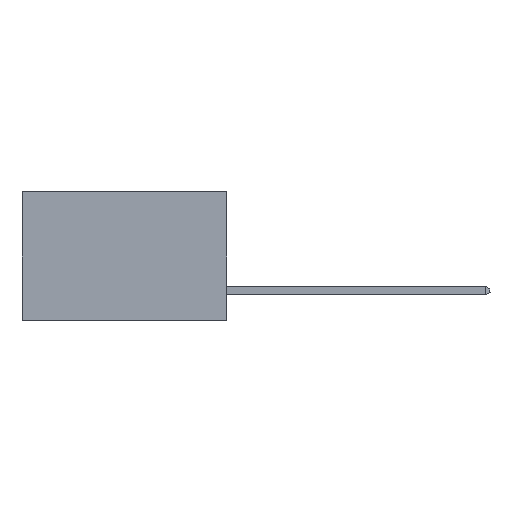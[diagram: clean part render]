
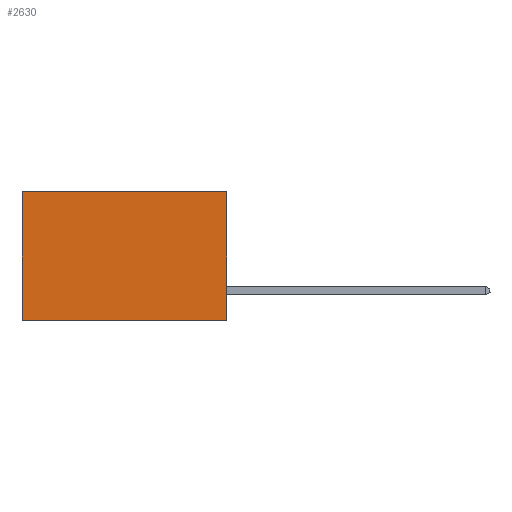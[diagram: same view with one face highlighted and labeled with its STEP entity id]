
A CAD part, left-side view. The second image highlights one B-rep face of the part: STEP entity #2630.
In plain terms, the highlighted planar face has unit normal (-1, 0, 0).
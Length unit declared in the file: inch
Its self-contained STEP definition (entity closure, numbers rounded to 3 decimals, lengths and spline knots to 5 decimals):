
#65 = DIRECTION ( 'NONE',  ( 0., 0., -1. ) ) ;
#293 = VECTOR ( 'NONE', #6475, 39.37008 ) ;
#1515 = AXIS2_PLACEMENT_3D ( 'NONE', #18451, #18292, #18211 ) ;
#2630 = ADVANCED_FACE ( 'NONE', ( #3477 ), #18608, .F. ) ;
#3477 = FACE_OUTER_BOUND ( 'NONE', #9012, .T. ) ;
#3936 = VERTEX_POINT ( 'NONE', #11721 ) ;
#5675 = LINE ( 'NONE', #19321, #19999 ) ;
#6475 = DIRECTION ( 'NONE',  ( 0., 1., 0. ) ) ;
#8043 = CARTESIAN_POINT ( 'NONE',  ( 0.277, 0., -0.37 ) ) ;
#8139 = DIRECTION ( 'NONE',  ( 0., 0., -1. ) ) ;
#8592 = VERTEX_POINT ( 'NONE', #22757 ) ;
#9012 = EDGE_LOOP ( 'NONE', ( #22453, #22119, #9803, #23677 ) ) ;
#9803 = ORIENTED_EDGE ( 'NONE', *, *, #16976, .F. ) ;
#10409 = LINE ( 'NONE', #23288, #293 ) ;
#11721 = CARTESIAN_POINT ( 'NONE',  ( 0.277, 0.59, 0. ) ) ;
#12514 = CARTESIAN_POINT ( 'NONE',  ( 0.277, 0., -0.37 ) ) ;
#15147 = VECTOR ( 'NONE', #8139, 39.37008 ) ;
#16976 = EDGE_CURVE ( 'NONE', #19534, #21288, #20615, .T. ) ;
#18064 = EDGE_CURVE ( 'NONE', #19534, #3936, #5675, .T. ) ;
#18211 = DIRECTION ( 'NONE',  ( 0., 0., -1. ) ) ;
#18292 = DIRECTION ( 'NONE',  ( 1., 0., 0. ) ) ;
#18451 = CARTESIAN_POINT ( 'NONE',  ( 0.277, 0., -0.37 ) ) ;
#18608 = PLANE ( 'NONE',  #1515 ) ;
#18717 = EDGE_CURVE ( 'NONE', #21288, #8592, #10409, .T. ) ;
#19321 = CARTESIAN_POINT ( 'NONE',  ( 0.277, 0., 0. ) ) ;
#19534 = VERTEX_POINT ( 'NONE', #23763 ) ;
#19919 = VECTOR ( 'NONE', #65, 39.37008 ) ;
#19999 = VECTOR ( 'NONE', #21204, 39.37008 ) ;
#20518 = LINE ( 'NONE', #22535, #19919 ) ;
#20615 = LINE ( 'NONE', #8043, #15147 ) ;
#21204 = DIRECTION ( 'NONE',  ( 0., 1., 0. ) ) ;
#21288 = VERTEX_POINT ( 'NONE', #12514 ) ;
#22119 = ORIENTED_EDGE ( 'NONE', *, *, #18717, .F. ) ;
#22126 = EDGE_CURVE ( 'NONE', #3936, #8592, #20518, .T. ) ;
#22453 = ORIENTED_EDGE ( 'NONE', *, *, #22126, .T. ) ;
#22535 = CARTESIAN_POINT ( 'NONE',  ( 0.277, 0.59, -0.37 ) ) ;
#22757 = CARTESIAN_POINT ( 'NONE',  ( 0.277, 0.59, -0.37 ) ) ;
#23288 = CARTESIAN_POINT ( 'NONE',  ( 0.277, 0., -0.37 ) ) ;
#23677 = ORIENTED_EDGE ( 'NONE', *, *, #18064, .T. ) ;
#23763 = CARTESIAN_POINT ( 'NONE',  ( 0.277, 0., 0. ) ) ;
